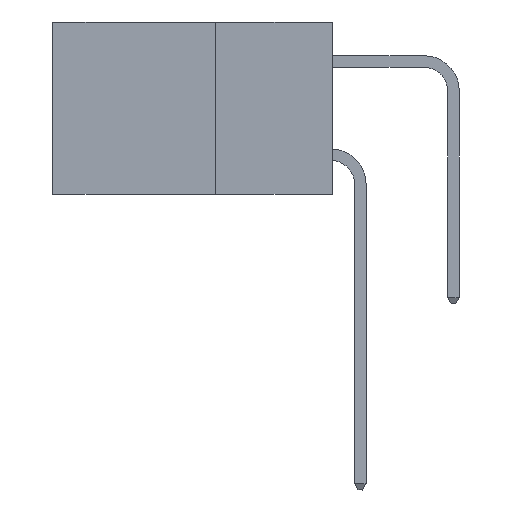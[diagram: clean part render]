
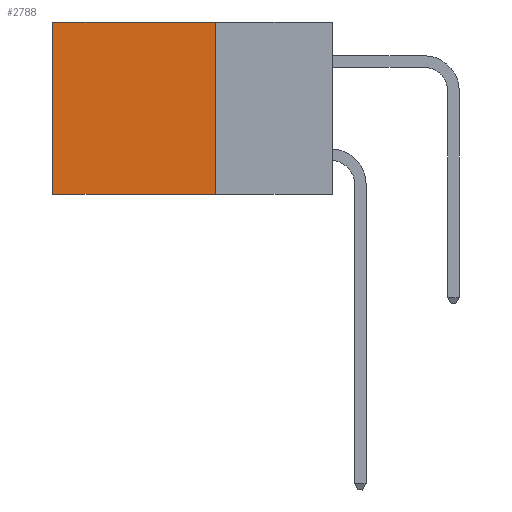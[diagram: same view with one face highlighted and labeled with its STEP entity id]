
A CAD part, left-side view. The second image highlights one B-rep face of the part: STEP entity #2788.
In plain terms, the highlighted planar face has unit normal (-1, 0, 0).
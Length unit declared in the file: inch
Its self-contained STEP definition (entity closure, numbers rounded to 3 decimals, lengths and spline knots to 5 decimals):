
#1141 = CARTESIAN_POINT ( 'NONE',  ( 0.2615, 0.25, -0.37 ) ) ;
#1482 = CARTESIAN_POINT ( 'NONE',  ( 0.2615, 0.25, -0.37 ) ) ;
#1632 = CARTESIAN_POINT ( 'NONE',  ( 0.2615, 0.25, 0. ) ) ;
#2520 = LINE ( 'NONE', #11246, #13806 ) ;
#2602 = ORIENTED_EDGE ( 'NONE', *, *, #7027, .T. ) ;
#2788 = ADVANCED_FACE ( 'NONE', ( #10743 ), #5150, .F. ) ;
#4286 = VERTEX_POINT ( 'NONE', #1141 ) ;
#4394 = ORIENTED_EDGE ( 'NONE', *, *, #8996, .F. ) ;
#4464 = EDGE_LOOP ( 'NONE', ( #5025, #10102, #4394, #2602 ) ) ;
#5000 = CARTESIAN_POINT ( 'NONE',  ( 0.2615, 0.25, 0. ) ) ;
#5025 = ORIENTED_EDGE ( 'NONE', *, *, #12325, .T. ) ;
#5150 = PLANE ( 'NONE',  #11170 ) ;
#6524 = VECTOR ( 'NONE', #8476, 39.37008 ) ;
#6615 = VERTEX_POINT ( 'NONE', #12770 ) ;
#6941 = VERTEX_POINT ( 'NONE', #8092 ) ;
#7027 = EDGE_CURVE ( 'NONE', #7049, #6615, #11927, .T. ) ;
#7049 = VERTEX_POINT ( 'NONE', #1632 ) ;
#8092 = CARTESIAN_POINT ( 'NONE',  ( 0.2615, 0.6, -0.37 ) ) ;
#8423 = VECTOR ( 'NONE', #8748, 39.37008 ) ;
#8476 = DIRECTION ( 'NONE',  ( 0., 1., 0. ) ) ;
#8748 = DIRECTION ( 'NONE',  ( 0., 0., -1. ) ) ;
#8996 = EDGE_CURVE ( 'NONE', #7049, #4286, #12504, .T. ) ;
#9643 = CARTESIAN_POINT ( 'NONE',  ( 0.2615, 0.25, -0.37 ) ) ;
#9881 = LINE ( 'NONE', #14335, #8423 ) ;
#10102 = ORIENTED_EDGE ( 'NONE', *, *, #11995, .F. ) ;
#10163 = DIRECTION ( 'NONE',  ( 0., 1., 0. ) ) ;
#10743 = FACE_OUTER_BOUND ( 'NONE', #4464, .T. ) ;
#11170 = AXIS2_PLACEMENT_3D ( 'NONE', #9643, #14111, #12887 ) ;
#11246 = CARTESIAN_POINT ( 'NONE',  ( 0.2615, 0.25, -0.37 ) ) ;
#11312 = DIRECTION ( 'NONE',  ( 0., 0., -1. ) ) ;
#11927 = LINE ( 'NONE', #5000, #6524 ) ;
#11995 = EDGE_CURVE ( 'NONE', #4286, #6941, #2520, .T. ) ;
#12325 = EDGE_CURVE ( 'NONE', #6615, #6941, #9881, .T. ) ;
#12504 = LINE ( 'NONE', #1482, #14206 ) ;
#12770 = CARTESIAN_POINT ( 'NONE',  ( 0.2615, 0.6, 0. ) ) ;
#12887 = DIRECTION ( 'NONE',  ( 0., 0., -1. ) ) ;
#13806 = VECTOR ( 'NONE', #10163, 39.37008 ) ;
#14111 = DIRECTION ( 'NONE',  ( 1., 0., 0. ) ) ;
#14206 = VECTOR ( 'NONE', #11312, 39.37008 ) ;
#14335 = CARTESIAN_POINT ( 'NONE',  ( 0.2615, 0.6, -0.37 ) ) ;
